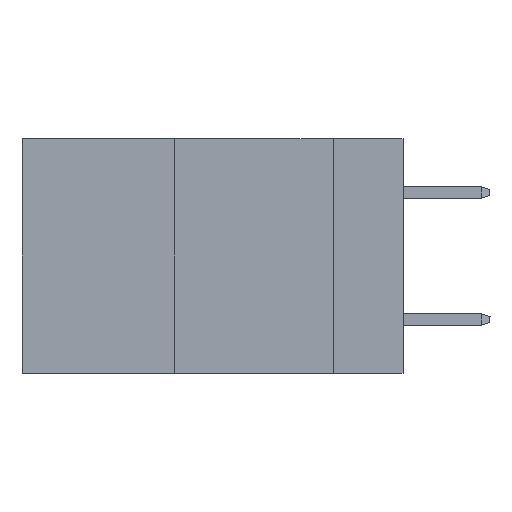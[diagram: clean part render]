
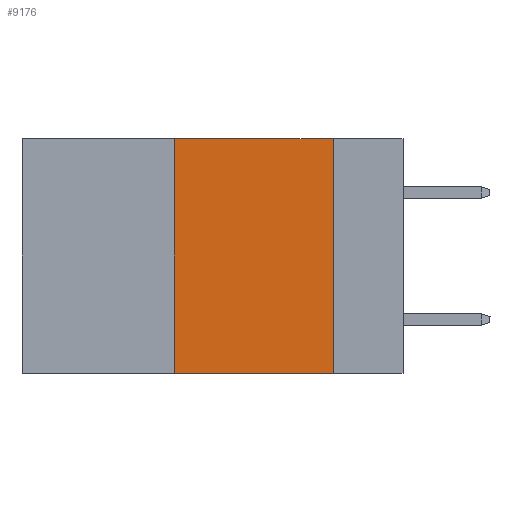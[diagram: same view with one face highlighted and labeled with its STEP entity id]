
A CAD part, left-side view. The second image highlights one B-rep face of the part: STEP entity #9176.
In plain terms, the highlighted planar face has unit normal (-1, 0, 0).
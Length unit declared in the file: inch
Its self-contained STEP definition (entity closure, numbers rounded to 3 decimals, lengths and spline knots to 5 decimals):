
#352 = EDGE_LOOP ( 'NONE', ( #8216, #13763, #18213, #13161 ) ) ;
#621 = VECTOR ( 'NONE', #6828, 39.37008 ) ;
#715 = VERTEX_POINT ( 'NONE', #14405 ) ;
#850 = CARTESIAN_POINT ( 'NONE',  ( 0., 0.36, 0. ) ) ;
#3384 = VERTEX_POINT ( 'NONE', #14205 ) ;
#3526 = LINE ( 'NONE', #5104, #621 ) ;
#3717 = EDGE_CURVE ( 'NONE', #715, #8047, #15227, .T. ) ;
#4936 = FACE_OUTER_BOUND ( 'NONE', #352, .T. ) ;
#5104 = CARTESIAN_POINT ( 'NONE',  ( 0., 0.6, -0.37 ) ) ;
#5511 = EDGE_CURVE ( 'NONE', #3384, #13429, #17317, .T. ) ;
#6020 = CARTESIAN_POINT ( 'NONE',  ( 0., 0.11, 0. ) ) ;
#6172 = DIRECTION ( 'NONE',  ( 1., 0., 0. ) ) ;
#6425 = AXIS2_PLACEMENT_3D ( 'NONE', #15168, #6172, #10814 ) ;
#6494 = EDGE_CURVE ( 'NONE', #8047, #3384, #17618, .T. ) ;
#6828 = DIRECTION ( 'NONE',  ( 0., -1., 0. ) ) ;
#7124 = VECTOR ( 'NONE', #13057, 39.37008 ) ;
#7723 = VECTOR ( 'NONE', #12082, 39.37008 ) ;
#8047 = VERTEX_POINT ( 'NONE', #850 ) ;
#8216 = ORIENTED_EDGE ( 'NONE', *, *, #5511, .F. ) ;
#8803 = CARTESIAN_POINT ( 'NONE',  ( 0., 0.6, 0. ) ) ;
#9176 = ADVANCED_FACE ( 'NONE', ( #4936 ), #16394, .F. ) ;
#9452 = CARTESIAN_POINT ( 'NONE',  ( 0., 0.36, 0. ) ) ;
#10814 = DIRECTION ( 'NONE',  ( 0., 0., -1. ) ) ;
#10953 = VECTOR ( 'NONE', #18746, 39.37008 ) ;
#12082 = DIRECTION ( 'NONE',  ( 0., 0., 1. ) ) ;
#12588 = EDGE_CURVE ( 'NONE', #715, #13429, #3526, .T. ) ;
#13057 = DIRECTION ( 'NONE',  ( 0., -1., 0. ) ) ;
#13161 = ORIENTED_EDGE ( 'NONE', *, *, #12588, .T. ) ;
#13429 = VERTEX_POINT ( 'NONE', #17102 ) ;
#13763 = ORIENTED_EDGE ( 'NONE', *, *, #6494, .F. ) ;
#14205 = CARTESIAN_POINT ( 'NONE',  ( 0., 0.11, 0. ) ) ;
#14405 = CARTESIAN_POINT ( 'NONE',  ( 0., 0.36, -0.37 ) ) ;
#15168 = CARTESIAN_POINT ( 'NONE',  ( 0., 0.6, 0. ) ) ;
#15227 = LINE ( 'NONE', #9452, #7723 ) ;
#16394 = PLANE ( 'NONE',  #6425 ) ;
#17102 = CARTESIAN_POINT ( 'NONE',  ( 0., 0.11, -0.37 ) ) ;
#17317 = LINE ( 'NONE', #6020, #10953 ) ;
#17618 = LINE ( 'NONE', #8803, #7124 ) ;
#18213 = ORIENTED_EDGE ( 'NONE', *, *, #3717, .F. ) ;
#18746 = DIRECTION ( 'NONE',  ( 0., 0., -1. ) ) ;
